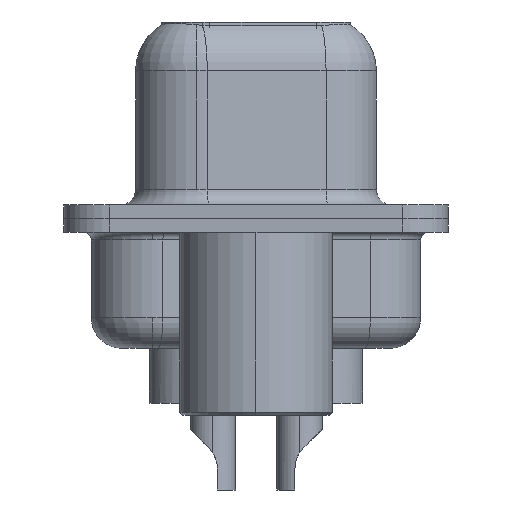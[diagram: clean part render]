
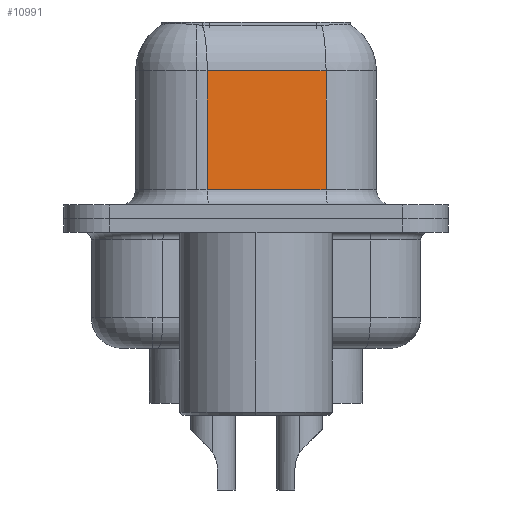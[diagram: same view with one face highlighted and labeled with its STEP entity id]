
A CAD part, left-side view. The second image highlights one B-rep face of the part: STEP entity #10991.
In plain terms, the highlighted planar face has unit normal (-0.985, -0.174, 0).
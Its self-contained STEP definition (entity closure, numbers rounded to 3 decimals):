
#58 = DIRECTION ( 'NONE',  ( 0., 0., -1. ) ) ;
#2511 = VECTOR ( 'NONE', #58, 1000. ) ;
#2988 = DIRECTION ( 'NONE',  ( 0., 0., -1. ) ) ;
#3054 = EDGE_CURVE ( 'NONE', #14538, #16031, #19379, .T. ) ;
#3258 = CARTESIAN_POINT ( 'NONE',  ( 5.063, -2.297, 6.6 ) ) ;
#3343 = VECTOR ( 'NONE', #2988, 1000. ) ;
#3402 = LINE ( 'NONE', #9804, #13232 ) ;
#4569 = VERTEX_POINT ( 'NONE', #13706 ) ;
#5395 = VERTEX_POINT ( 'NONE', #6050 ) ;
#5675 = DIRECTION ( 'NONE',  ( 0.174, -0.985, 0. ) ) ;
#6050 = CARTESIAN_POINT ( 'NONE',  ( 5.063, -2.297, 4.85 ) ) ;
#7483 = LINE ( 'NONE', #12109, #3343 ) ;
#7555 = PLANE ( 'NONE',  #13062 ) ;
#8787 = CARTESIAN_POINT ( 'NONE',  ( 5.063, -2.297, 0.95 ) ) ;
#9149 = LINE ( 'NONE', #18538, #2511 ) ;
#9356 = FACE_OUTER_BOUND ( 'NONE', #19695, .T. ) ;
#9418 = CARTESIAN_POINT ( 'NONE',  ( 4.375, 1.603, 0.95 ) ) ;
#9804 = CARTESIAN_POINT ( 'NONE',  ( 5.063, -2.297, 4.85 ) ) ;
#10991 = ADVANCED_FACE ( 'NONE', ( #9356 ), #7555, .F. ) ;
#11016 = CARTESIAN_POINT ( 'NONE',  ( 5.063, -2.297, 0.95 ) ) ;
#11212 = DIRECTION ( 'NONE',  ( -0.174, 0.985, 0. ) ) ;
#12109 = CARTESIAN_POINT ( 'NONE',  ( 4.375, 1.603, 6.6 ) ) ;
#12643 = EDGE_CURVE ( 'NONE', #5395, #16031, #9149, .T. ) ;
#12788 = ORIENTED_EDGE ( 'NONE', *, *, #16006, .T. ) ;
#13062 = AXIS2_PLACEMENT_3D ( 'NONE', #3258, #13878, #15471 ) ;
#13232 = VECTOR ( 'NONE', #11212, 1000. ) ;
#13646 = EDGE_CURVE ( 'NONE', #4569, #14538, #7483, .T. ) ;
#13706 = CARTESIAN_POINT ( 'NONE',  ( 4.375, 1.603, 4.85 ) ) ;
#13878 = DIRECTION ( 'NONE',  ( 0.985, 0.174, 0. ) ) ;
#14538 = VERTEX_POINT ( 'NONE', #9418 ) ;
#14872 = ORIENTED_EDGE ( 'NONE', *, *, #12643, .F. ) ;
#15471 = DIRECTION ( 'NONE',  ( -0.174, 0.985, 0. ) ) ;
#16006 = EDGE_CURVE ( 'NONE', #5395, #4569, #3402, .T. ) ;
#16031 = VERTEX_POINT ( 'NONE', #11016 ) ;
#17078 = ORIENTED_EDGE ( 'NONE', *, *, #13646, .T. ) ;
#18538 = CARTESIAN_POINT ( 'NONE',  ( 5.063, -2.297, 6.6 ) ) ;
#19028 = VECTOR ( 'NONE', #5675, 1000. ) ;
#19277 = ORIENTED_EDGE ( 'NONE', *, *, #3054, .T. ) ;
#19379 = LINE ( 'NONE', #8787, #19028 ) ;
#19695 = EDGE_LOOP ( 'NONE', ( #14872, #12788, #17078, #19277 ) ) ;
